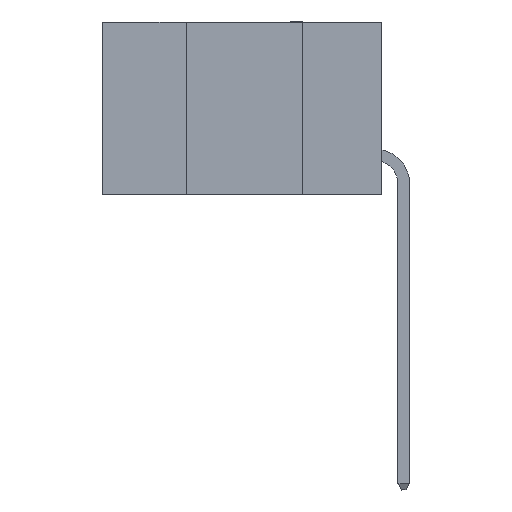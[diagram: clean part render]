
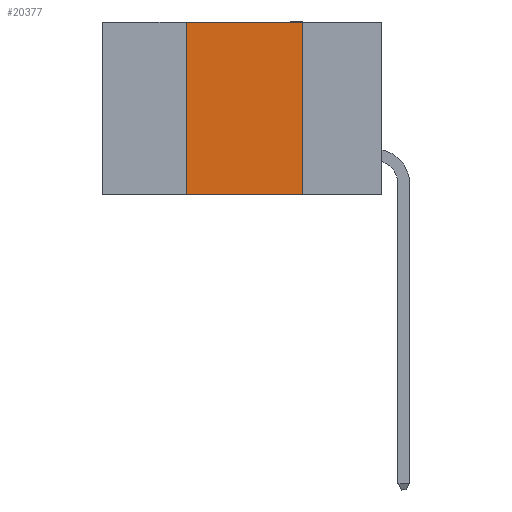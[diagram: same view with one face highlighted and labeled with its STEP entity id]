
A CAD part, left-side view. The second image highlights one B-rep face of the part: STEP entity #20377.
In plain terms, the highlighted planar face has unit normal (-1, 0, 0).
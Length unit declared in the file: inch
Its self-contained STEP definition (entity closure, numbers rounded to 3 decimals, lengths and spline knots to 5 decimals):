
#196 = EDGE_LOOP ( 'NONE', ( #820, #13328, #246, #27845 ) ) ;
#246 = ORIENTED_EDGE ( 'NONE', *, *, #28761, .F. ) ;
#820 = ORIENTED_EDGE ( 'NONE', *, *, #1090, .F. ) ;
#1090 = EDGE_CURVE ( 'NONE', #6400, #21145, #28568, .T. ) ;
#1636 = CARTESIAN_POINT ( 'NONE',  ( 0., 0.42, -0.37 ) ) ;
#2333 = LINE ( 'NONE', #20980, #9725 ) ;
#3671 = VECTOR ( 'NONE', #27292, 39.37008 ) ;
#4026 = LINE ( 'NONE', #28657, #3671 ) ;
#4547 = VECTOR ( 'NONE', #6845, 39.37008 ) ;
#5286 = PLANE ( 'NONE',  #12575 ) ;
#5306 = LINE ( 'NONE', #14856, #24880 ) ;
#5808 = CARTESIAN_POINT ( 'NONE',  ( 0., 0.17, -0.37 ) ) ;
#6008 = DIRECTION ( 'NONE',  ( 1., 0., 0. ) ) ;
#6384 = EDGE_CURVE ( 'NONE', #15247, #6400, #5306, .T. ) ;
#6400 = VERTEX_POINT ( 'NONE', #23675 ) ;
#6845 = DIRECTION ( 'NONE',  ( 0., 0., -1. ) ) ;
#9725 = VECTOR ( 'NONE', #21177, 39.37008 ) ;
#10666 = CARTESIAN_POINT ( 'NONE',  ( 0., 0.6, 0. ) ) ;
#12575 = AXIS2_PLACEMENT_3D ( 'NONE', #10666, #6008, #19689 ) ;
#13328 = ORIENTED_EDGE ( 'NONE', *, *, #6384, .F. ) ;
#13704 = EDGE_CURVE ( 'NONE', #26843, #21145, #4026, .T. ) ;
#14856 = CARTESIAN_POINT ( 'NONE',  ( 0., 0.6, 0. ) ) ;
#15247 = VERTEX_POINT ( 'NONE', #23438 ) ;
#17182 = DIRECTION ( 'NONE',  ( 0., -1., 0. ) ) ;
#18545 = CARTESIAN_POINT ( 'NONE',  ( 0., 0.17, 0. ) ) ;
#19689 = DIRECTION ( 'NONE',  ( 0., 0., -1. ) ) ;
#20377 = ADVANCED_FACE ( 'NONE', ( #27819 ), #5286, .F. ) ;
#20980 = CARTESIAN_POINT ( 'NONE',  ( 0., 0.42, 0. ) ) ;
#21145 = VERTEX_POINT ( 'NONE', #5808 ) ;
#21177 = DIRECTION ( 'NONE',  ( 0., 0., 1. ) ) ;
#23438 = CARTESIAN_POINT ( 'NONE',  ( 0., 0.42, 0. ) ) ;
#23675 = CARTESIAN_POINT ( 'NONE',  ( 0., 0.17, 0. ) ) ;
#24880 = VECTOR ( 'NONE', #17182, 39.37008 ) ;
#26843 = VERTEX_POINT ( 'NONE', #1636 ) ;
#27292 = DIRECTION ( 'NONE',  ( 0., -1., 0. ) ) ;
#27819 = FACE_OUTER_BOUND ( 'NONE', #196, .T. ) ;
#27845 = ORIENTED_EDGE ( 'NONE', *, *, #13704, .T. ) ;
#28568 = LINE ( 'NONE', #18545, #4547 ) ;
#28657 = CARTESIAN_POINT ( 'NONE',  ( 0., 0.6, -0.37 ) ) ;
#28761 = EDGE_CURVE ( 'NONE', #26843, #15247, #2333, .T. ) ;
